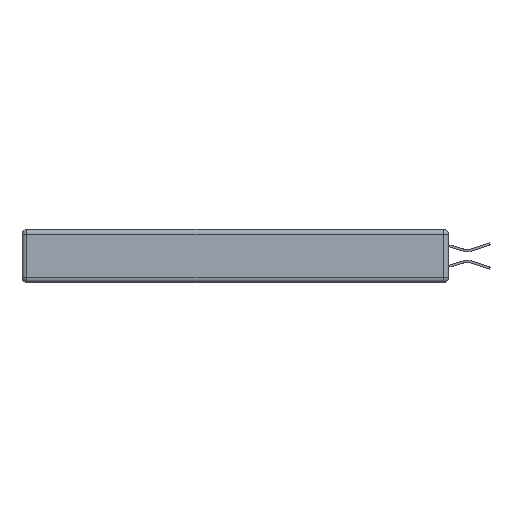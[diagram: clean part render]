
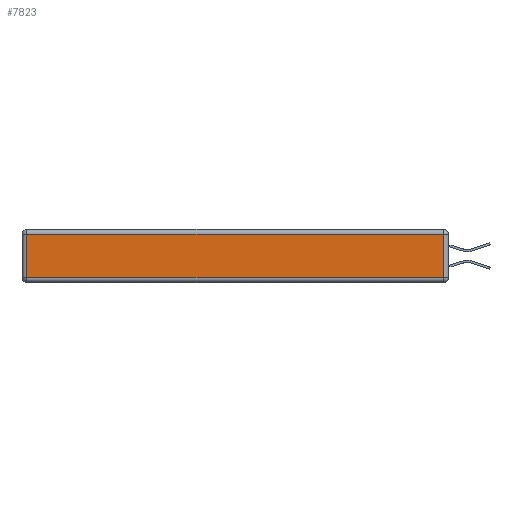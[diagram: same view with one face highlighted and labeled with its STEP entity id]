
A CAD part, left-side view. The second image highlights one B-rep face of the part: STEP entity #7823.
In plain terms, the highlighted planar face has unit normal (-1, 0, 0).
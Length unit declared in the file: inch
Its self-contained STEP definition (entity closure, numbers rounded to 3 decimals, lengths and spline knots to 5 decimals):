
#379 = FACE_OUTER_BOUND ( 'NONE', #16737, .T. ) ;
#438 = PLANE ( 'NONE',  #8603 ) ;
#581 = DIRECTION ( 'NONE',  ( 0., 1., 0. ) ) ;
#1438 = CARTESIAN_POINT ( 'NONE',  ( 0., 0.03, -0.03 ) ) ;
#1790 = DIRECTION ( 'NONE',  ( -1., 0., 0. ) ) ;
#1918 = DIRECTION ( 'NONE',  ( 0., 0., 1. ) ) ;
#2631 = EDGE_CURVE ( 'NONE', #6727, #6404, #3377, .T. ) ;
#2781 = CARTESIAN_POINT ( 'NONE',  ( 0., 0., -0.313 ) ) ;
#3273 = VECTOR ( 'NONE', #5390, 39.37008 ) ;
#3377 = LINE ( 'NONE', #6009, #9008 ) ;
#3506 = CARTESIAN_POINT ( 'NONE',  ( 0., 0.03, -0.313 ) ) ;
#4053 = CARTESIAN_POINT ( 'NONE',  ( 0., 2.72, -0.343 ) ) ;
#4059 = CARTESIAN_POINT ( 'NONE',  ( 0., 2.72, -0.03 ) ) ;
#4628 = EDGE_CURVE ( 'NONE', #9589, #6727, #17287, .T. ) ;
#4645 = CARTESIAN_POINT ( 'NONE',  ( 0., 0., -0.343 ) ) ;
#4959 = EDGE_CURVE ( 'NONE', #16313, #9589, #10684, .T. ) ;
#5390 = DIRECTION ( 'NONE',  ( 0., -1., 0. ) ) ;
#5721 = CARTESIAN_POINT ( 'NONE',  ( 0., 2.72, -0.313 ) ) ;
#5936 = DIRECTION ( 'NONE',  ( 0., 0., 1. ) ) ;
#6009 = CARTESIAN_POINT ( 'NONE',  ( 0., 2.75, -0.03 ) ) ;
#6404 = VERTEX_POINT ( 'NONE', #4059 ) ;
#6727 = VERTEX_POINT ( 'NONE', #1438 ) ;
#7823 = ADVANCED_FACE ( 'NONE', ( #379 ), #438, .T. ) ;
#8420 = ORIENTED_EDGE ( 'NONE', *, *, #4959, .T. ) ;
#8480 = VECTOR ( 'NONE', #17988, 39.37008 ) ;
#8603 = AXIS2_PLACEMENT_3D ( 'NONE', #4645, #1790, #1918 ) ;
#9008 = VECTOR ( 'NONE', #581, 39.37008 ) ;
#9589 = VERTEX_POINT ( 'NONE', #3506 ) ;
#10684 = LINE ( 'NONE', #2781, #3273 ) ;
#11388 = ORIENTED_EDGE ( 'NONE', *, *, #2631, .T. ) ;
#11706 = ORIENTED_EDGE ( 'NONE', *, *, #13432, .T. ) ;
#12862 = ORIENTED_EDGE ( 'NONE', *, *, #4628, .T. ) ;
#13432 = EDGE_CURVE ( 'NONE', #6404, #16313, #17230, .T. ) ;
#15536 = VECTOR ( 'NONE', #5936, 39.37008 ) ;
#15616 = CARTESIAN_POINT ( 'NONE',  ( 0., 0.03, -0.343 ) ) ;
#16313 = VERTEX_POINT ( 'NONE', #5721 ) ;
#16737 = EDGE_LOOP ( 'NONE', ( #8420, #12862, #11388, #11706 ) ) ;
#17230 = LINE ( 'NONE', #4053, #8480 ) ;
#17287 = LINE ( 'NONE', #15616, #15536 ) ;
#17988 = DIRECTION ( 'NONE',  ( 0., 0., -1. ) ) ;
